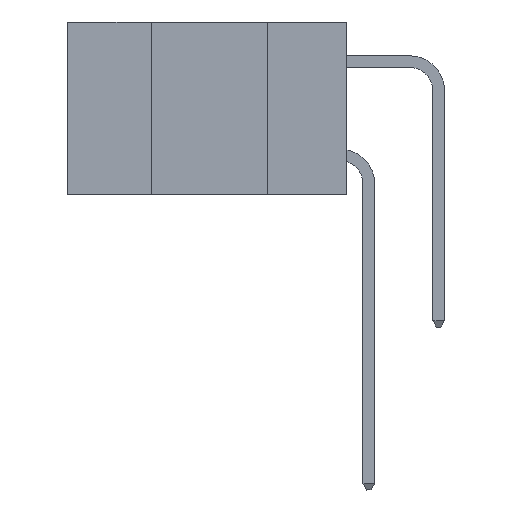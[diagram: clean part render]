
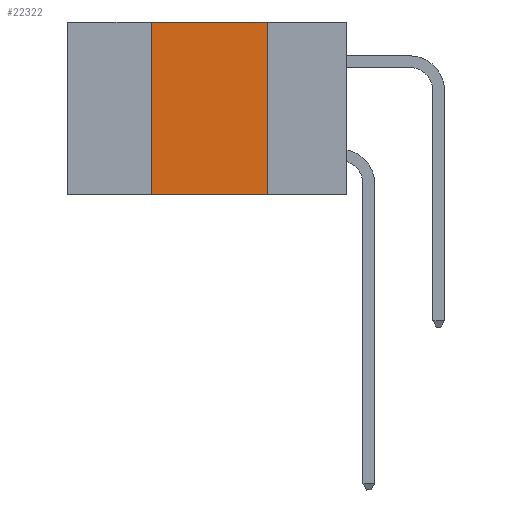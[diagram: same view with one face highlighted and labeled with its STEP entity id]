
A CAD part, left-side view. The second image highlights one B-rep face of the part: STEP entity #22322.
In plain terms, the highlighted planar face has unit normal (-1, 0, 0).
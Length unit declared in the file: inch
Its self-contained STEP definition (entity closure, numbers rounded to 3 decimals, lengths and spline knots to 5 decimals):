
#668 = VERTEX_POINT ( 'NONE', #13405 ) ;
#671 = CARTESIAN_POINT ( 'NONE',  ( 0., 0.6, 0. ) ) ;
#1173 = FACE_OUTER_BOUND ( 'NONE', #23304, .T. ) ;
#1695 = ORIENTED_EDGE ( 'NONE', *, *, #3623, .F. ) ;
#3623 = EDGE_CURVE ( 'NONE', #17905, #11073, #29435, .T. ) ;
#4567 = EDGE_CURVE ( 'NONE', #11073, #668, #24229, .T. ) ;
#5678 = DIRECTION ( 'NONE',  ( 0., 0., -1. ) ) ;
#7580 = CARTESIAN_POINT ( 'NONE',  ( 0., 0.42, 0. ) ) ;
#9329 = CARTESIAN_POINT ( 'NONE',  ( 0., 0.17, -0.37 ) ) ;
#10174 = DIRECTION ( 'NONE',  ( 0., 0., -1. ) ) ;
#11073 = VERTEX_POINT ( 'NONE', #23872 ) ;
#12500 = CARTESIAN_POINT ( 'NONE',  ( 0., 0.17, 0. ) ) ;
#12712 = EDGE_CURVE ( 'NONE', #668, #18244, #24277, .T. ) ;
#13253 = EDGE_CURVE ( 'NONE', #17905, #18244, #20189, .T. ) ;
#13277 = CARTESIAN_POINT ( 'NONE',  ( 0., 0.6, 0. ) ) ;
#13405 = CARTESIAN_POINT ( 'NONE',  ( 0., 0.17, 0. ) ) ;
#14707 = DIRECTION ( 'NONE',  ( 0., 0., 1. ) ) ;
#17756 = PLANE ( 'NONE',  #28685 ) ;
#17905 = VERTEX_POINT ( 'NONE', #19848 ) ;
#18244 = VERTEX_POINT ( 'NONE', #9329 ) ;
#18348 = ORIENTED_EDGE ( 'NONE', *, *, #13253, .T. ) ;
#19848 = CARTESIAN_POINT ( 'NONE',  ( 0., 0.42, -0.37 ) ) ;
#20070 = DIRECTION ( 'NONE',  ( 1., 0., 0. ) ) ;
#20189 = LINE ( 'NONE', #27026, #26567 ) ;
#22049 = DIRECTION ( 'NONE',  ( 0., -1., 0. ) ) ;
#22322 = ADVANCED_FACE ( 'NONE', ( #1173 ), #17756, .F. ) ;
#22586 = ORIENTED_EDGE ( 'NONE', *, *, #12712, .F. ) ;
#23304 = EDGE_LOOP ( 'NONE', ( #22586, #28323, #1695, #18348 ) ) ;
#23872 = CARTESIAN_POINT ( 'NONE',  ( 0., 0.42, 0. ) ) ;
#24229 = LINE ( 'NONE', #671, #25144 ) ;
#24277 = LINE ( 'NONE', #12500, #26538 ) ;
#24840 = DIRECTION ( 'NONE',  ( 0., -1., 0. ) ) ;
#25144 = VECTOR ( 'NONE', #22049, 39.37008 ) ;
#26514 = VECTOR ( 'NONE', #14707, 39.37008 ) ;
#26538 = VECTOR ( 'NONE', #5678, 39.37008 ) ;
#26567 = VECTOR ( 'NONE', #24840, 39.37008 ) ;
#27026 = CARTESIAN_POINT ( 'NONE',  ( 0., 0.6, -0.37 ) ) ;
#28323 = ORIENTED_EDGE ( 'NONE', *, *, #4567, .F. ) ;
#28685 = AXIS2_PLACEMENT_3D ( 'NONE', #13277, #20070, #10174 ) ;
#29435 = LINE ( 'NONE', #7580, #26514 ) ;
